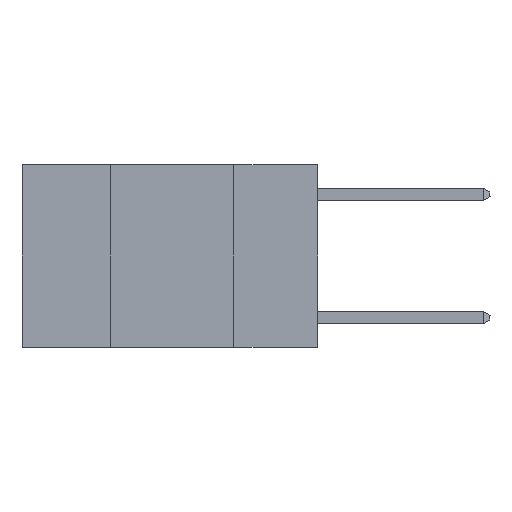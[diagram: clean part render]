
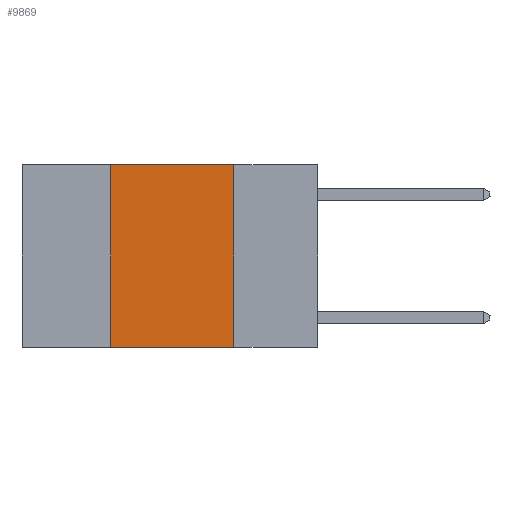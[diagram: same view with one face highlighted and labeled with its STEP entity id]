
A CAD part, left-side view. The second image highlights one B-rep face of the part: STEP entity #9869.
In plain terms, the highlighted planar face has unit normal (-1, 0, 0).
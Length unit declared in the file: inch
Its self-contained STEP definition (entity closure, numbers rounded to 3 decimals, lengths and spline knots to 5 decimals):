
#710 = PLANE ( 'NONE',  #9776 ) ;
#760 = ORIENTED_EDGE ( 'NONE', *, *, #10008, .T. ) ;
#1240 = DIRECTION ( 'NONE',  ( 0., 0., 1. ) ) ;
#1581 = FACE_OUTER_BOUND ( 'NONE', #3288, .T. ) ;
#1635 = CARTESIAN_POINT ( 'NONE',  ( 0., 0.17, -0.37 ) ) ;
#1810 = CARTESIAN_POINT ( 'NONE',  ( 0., 0.6, 0. ) ) ;
#1845 = VERTEX_POINT ( 'NONE', #1635 ) ;
#1874 = DIRECTION ( 'NONE',  ( 0., 0., -1. ) ) ;
#1968 = DIRECTION ( 'NONE',  ( 1., 0., 0. ) ) ;
#2032 = CARTESIAN_POINT ( 'NONE',  ( 0., 0.17, 0. ) ) ;
#3288 = EDGE_LOOP ( 'NONE', ( #4050, #9021, #8755, #760 ) ) ;
#3289 = CARTESIAN_POINT ( 'NONE',  ( 0., 0.17, 0. ) ) ;
#3495 = VERTEX_POINT ( 'NONE', #10619 ) ;
#4050 = ORIENTED_EDGE ( 'NONE', *, *, #10455, .F. ) ;
#4716 = CARTESIAN_POINT ( 'NONE',  ( 0., 0.6, -0.37 ) ) ;
#4773 = LINE ( 'NONE', #4716, #9606 ) ;
#4774 = DIRECTION ( 'NONE',  ( 0., 0., -1. ) ) ;
#4861 = CARTESIAN_POINT ( 'NONE',  ( 0., 0.6, 0. ) ) ;
#5501 = CARTESIAN_POINT ( 'NONE',  ( 0., 0.42, 0. ) ) ;
#5504 = LINE ( 'NONE', #2032, #6471 ) ;
#5774 = DIRECTION ( 'NONE',  ( 0., -1., 0. ) ) ;
#6471 = VECTOR ( 'NONE', #4774, 39.37008 ) ;
#7360 = VECTOR ( 'NONE', #5774, 39.37008 ) ;
#7822 = VERTEX_POINT ( 'NONE', #3289 ) ;
#8383 = LINE ( 'NONE', #4861, #7360 ) ;
#8496 = VERTEX_POINT ( 'NONE', #5501 ) ;
#8755 = ORIENTED_EDGE ( 'NONE', *, *, #9692, .F. ) ;
#9021 = ORIENTED_EDGE ( 'NONE', *, *, #9231, .F. ) ;
#9231 = EDGE_CURVE ( 'NONE', #8496, #7822, #8383, .T. ) ;
#9606 = VECTOR ( 'NONE', #10011, 39.37008 ) ;
#9692 = EDGE_CURVE ( 'NONE', #3495, #8496, #10984, .T. ) ;
#9776 = AXIS2_PLACEMENT_3D ( 'NONE', #1810, #1968, #1874 ) ;
#9869 = ADVANCED_FACE ( 'NONE', ( #1581 ), #710, .F. ) ;
#10008 = EDGE_CURVE ( 'NONE', #3495, #1845, #4773, .T. ) ;
#10011 = DIRECTION ( 'NONE',  ( 0., -1., 0. ) ) ;
#10023 = CARTESIAN_POINT ( 'NONE',  ( 0., 0.42, 0. ) ) ;
#10455 = EDGE_CURVE ( 'NONE', #7822, #1845, #5504, .T. ) ;
#10499 = VECTOR ( 'NONE', #1240, 39.37008 ) ;
#10619 = CARTESIAN_POINT ( 'NONE',  ( 0., 0.42, -0.37 ) ) ;
#10984 = LINE ( 'NONE', #10023, #10499 ) ;
